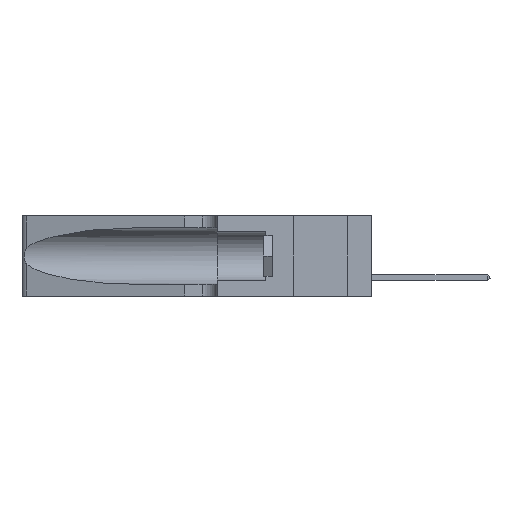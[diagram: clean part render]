
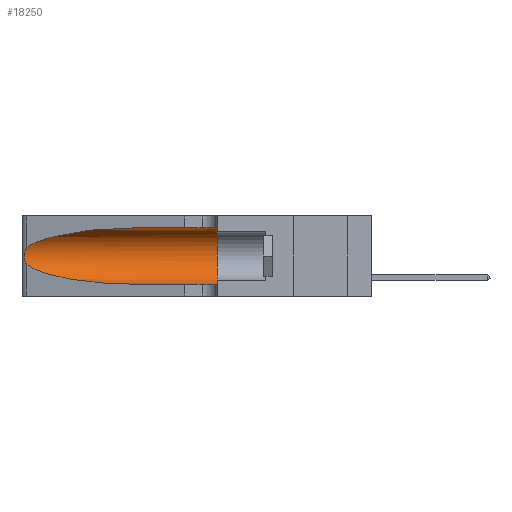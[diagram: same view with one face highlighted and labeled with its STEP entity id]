
A CAD part, left-side view. The second image highlights one B-rep face of the part: STEP entity #18250.
In plain terms, the highlighted cylindrical face has radius 3.308 mm (diameter 6.617 mm), a partial arc.
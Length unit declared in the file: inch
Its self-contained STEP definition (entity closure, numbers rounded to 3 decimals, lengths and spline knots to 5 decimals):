
#247 = CARTESIAN_POINT ( 'NONE',  ( 0.18966, 0.96281, 0.31525 ) ) ;
#454 = CARTESIAN_POINT ( 'NONE',  ( 0.25487, 1.22718, 0.22369 ) ) ;
#606 = CARTESIAN_POINT ( 'NONE',  ( 0.25487, 1.22718, 0.14631 ) ) ;
#670 = CARTESIAN_POINT ( 'NONE',  ( 0.1305, 0.35, 0.185 ) ) ;
#747 = LINE ( 'NONE', #1557, #12815 ) ;
#1088 = DIRECTION ( 'NONE',  ( 0., -1., 0. ) ) ;
#1557 = CARTESIAN_POINT ( 'NONE',  ( 0.1305, 1.61858, 0.05475 ) ) ;
#1636 = EDGE_CURVE ( 'NONE', #4232, #6280, #10866, .T. ) ;
#1869 = EDGE_CURVE ( 'NONE', #14631, #4232, #17302, .T. ) ;
#2037 = CARTESIAN_POINT ( 'NONE',  ( 0.26017, 1.23833, 0.17102 ) ) ;
#2114 = CARTESIAN_POINT ( 'NONE',  ( 0.25555, 1.22993, 0.14849 ) ) ;
#2460 = CARTESIAN_POINT ( 'NONE',  ( 0.1305, 0.72297, 0.31525 ) ) ;
#2717 = DIRECTION ( 'NONE',  ( 0., 0., 1. ) ) ;
#3119 = CARTESIAN_POINT ( 'NONE',  ( 0.1305, 0.72297, 0.05475 ) ) ;
#3254 = FACE_OUTER_BOUND ( 'NONE', #21449, .T. ) ;
#3379 = ORIENTED_EDGE ( 'NONE', *, *, #21634, .T. ) ;
#3831 = CIRCLE ( 'NONE', #15025, 0.13025 ) ;
#4185 = AXIS2_PLACEMENT_3D ( 'NONE', #11712, #1088, #11642 ) ;
#4232 = VERTEX_POINT ( 'NONE', #9228 ) ;
#5098 = ORIENTED_EDGE ( 'NONE', *, *, #12150, .T. ) ;
#5214 = DIRECTION ( 'NONE',  ( 0., -1., 0. ) ) ;
#5509 = CARTESIAN_POINT ( 'NONE',  ( 0.1305, 1.61858, 0.31525 ) ) ;
#5510 = CARTESIAN_POINT ( 'NONE',  ( 0.1305, 0.35, 0.31525 ) ) ;
#5563 = CARTESIAN_POINT ( 'NONE',  ( 0.25789, 1.23486, 0.15765 ) ) ;
#6280 = VERTEX_POINT ( 'NONE', #17986 ) ;
#7399 = CARTESIAN_POINT ( 'NONE',  ( 0.25639, 1.23184, 0.21858 ) ) ;
#7554 = CARTESIAN_POINT ( 'NONE',  ( 0.25854, 1.2359, 0.20912 ) ) ;
#8247 = CARTESIAN_POINT ( 'NONE',  ( 0.18966, 0.96281, 0.05475 ) ) ;
#9091 = CARTESIAN_POINT ( 'NONE',  ( 0.26075, 1.23896, 0.178 ) ) ;
#9228 = CARTESIAN_POINT ( 'NONE',  ( 0.25487, 1.22718, 0.14631 ) ) ;
#9596 =( BOUNDED_CURVE ( )  B_SPLINE_CURVE ( 3, ( #11027, #247, #21518, #16381 ),
 .UNSPECIFIED., .F., .T. ) 
 B_SPLINE_CURVE_WITH_KNOTS ( ( 4, 4 ),
 ( 1.5708, 2.84003 ),
 .UNSPECIFIED. ) 
 CURVE ( )  GEOMETRIC_REPRESENTATION_ITEM ( )  RATIONAL_B_SPLINE_CURVE ( ( 1., 0.87, 0.87, 1. ) ) 
 REPRESENTATION_ITEM ( '' )  );
#10124 = CYLINDRICAL_SURFACE ( 'NONE', #4185, 0.13025 ) ;
#10799 = CARTESIAN_POINT ( 'NONE',  ( 0.25555, 1.22994, 0.2215 ) ) ;
#10866 =( BOUNDED_CURVE ( )  B_SPLINE_CURVE ( 3, ( #18805, #22369, #8247, #3119 ),
 .UNSPECIFIED., .F., .F. ) 
 B_SPLINE_CURVE_WITH_KNOTS ( ( 4, 4 ),
 ( 3.44316, 4.71239 ),
 .UNSPECIFIED. ) 
 CURVE ( )  GEOMETRIC_REPRESENTATION_ITEM ( )  RATIONAL_B_SPLINE_CURVE ( ( 1., 0.87, 0.87, 1. ) ) 
 REPRESENTATION_ITEM ( '' )  );
#11027 = CARTESIAN_POINT ( 'NONE',  ( 0.1305, 0.72297, 0.31525 ) ) ;
#11642 = DIRECTION ( 'NONE',  ( 0., 0., -1. ) ) ;
#11645 = VERTEX_POINT ( 'NONE', #2460 ) ;
#11712 = CARTESIAN_POINT ( 'NONE',  ( 0.1305, 1.61858, 0.185 ) ) ;
#12150 = EDGE_CURVE ( 'NONE', #11645, #14631, #9596, .T. ) ;
#12287 = ORIENTED_EDGE ( 'NONE', *, *, #1636, .T. ) ;
#12604 = CARTESIAN_POINT ( 'NONE',  ( 0.1305, 0.35, 0.05475 ) ) ;
#12815 = VECTOR ( 'NONE', #5214, 39.37008 ) ;
#13104 = EDGE_CURVE ( 'NONE', #15319, #16562, #3831, .T. ) ;
#13237 = DIRECTION ( 'NONE',  ( 0., 1., 0. ) ) ;
#13914 = EDGE_CURVE ( 'NONE', #11645, #15319, #22263, .T. ) ;
#14631 = VERTEX_POINT ( 'NONE', #454 ) ;
#15025 = AXIS2_PLACEMENT_3D ( 'NONE', #670, #13237, #2717 ) ;
#15319 = VERTEX_POINT ( 'NONE', #5510 ) ;
#15509 = ORIENTED_EDGE ( 'NONE', *, *, #1869, .T. ) ;
#16084 = CARTESIAN_POINT ( 'NONE',  ( 0.26018, 1.23835, 0.19895 ) ) ;
#16373 = ORIENTED_EDGE ( 'NONE', *, *, #13914, .F. ) ;
#16381 = CARTESIAN_POINT ( 'NONE',  ( 0.25487, 1.22718, 0.22369 ) ) ;
#16562 = VERTEX_POINT ( 'NONE', #12604 ) ;
#17226 = VECTOR ( 'NONE', #17801, 39.37008 ) ;
#17302 = B_SPLINE_CURVE_WITH_KNOTS ( 'NONE', 3,
 ( #18085, #10799, #7399, #19643, #7554, #16084, #19561, #9091, #2037, #21362, #5563, #17851, #2114, #606 ),
 .UNSPECIFIED., .F., .F.,
 ( 4, 2, 2, 2, 2, 2, 4 ),
 ( 0., 0.00027, 0.00053, 0.00107, 0.0016, 0.00187, 0.00214 ),
 .UNSPECIFIED. ) ;
#17801 = DIRECTION ( 'NONE',  ( 0., -1., 0. ) ) ;
#17851 = CARTESIAN_POINT ( 'NONE',  ( 0.25639, 1.23186, 0.15144 ) ) ;
#17986 = CARTESIAN_POINT ( 'NONE',  ( 0.1305, 0.72297, 0.05475 ) ) ;
#18085 = CARTESIAN_POINT ( 'NONE',  ( 0.25487, 1.22718, 0.22369 ) ) ;
#18250 = ADVANCED_FACE ( 'NONE', ( #3254 ), #10124, .F. ) ;
#18805 = CARTESIAN_POINT ( 'NONE',  ( 0.25487, 1.22718, 0.14631 ) ) ;
#19561 = CARTESIAN_POINT ( 'NONE',  ( 0.26075, 1.23896, 0.19203 ) ) ;
#19643 = CARTESIAN_POINT ( 'NONE',  ( 0.25787, 1.23484, 0.2124 ) ) ;
#20767 = ORIENTED_EDGE ( 'NONE', *, *, #13104, .F. ) ;
#21362 = CARTESIAN_POINT ( 'NONE',  ( 0.25856, 1.23593, 0.16098 ) ) ;
#21449 = EDGE_LOOP ( 'NONE', ( #5098, #15509, #12287, #3379, #20767, #16373 ) ) ;
#21518 = CARTESIAN_POINT ( 'NONE',  ( 0.2373, 1.15595, 0.28018 ) ) ;
#21634 = EDGE_CURVE ( 'NONE', #6280, #16562, #747, .T. ) ;
#22263 = LINE ( 'NONE', #5509, #17226 ) ;
#22369 = CARTESIAN_POINT ( 'NONE',  ( 0.2373, 1.15595, 0.08982 ) ) ;
